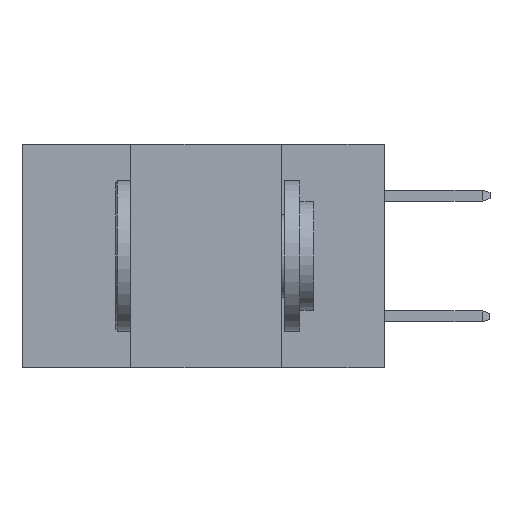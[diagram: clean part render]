
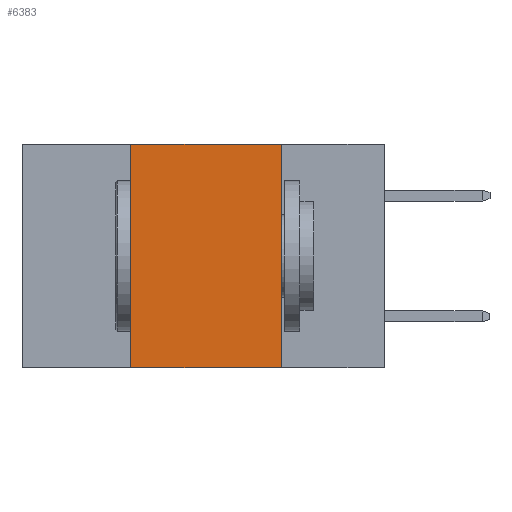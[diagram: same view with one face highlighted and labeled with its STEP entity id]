
A CAD part, left-side view. The second image highlights one B-rep face of the part: STEP entity #6383.
In plain terms, the highlighted planar face has unit normal (-1, 0, 0).
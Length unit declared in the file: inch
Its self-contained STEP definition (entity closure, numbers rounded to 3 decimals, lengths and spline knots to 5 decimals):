
#895 = CARTESIAN_POINT ( 'NONE',  ( 0., 0.17, 0. ) ) ;
#4665 = VECTOR ( 'NONE', #22252, 39.37008 ) ;
#5161 = EDGE_CURVE ( 'NONE', #11860, #26201, #27916, .T. ) ;
#5984 = CARTESIAN_POINT ( 'NONE',  ( 0., 0.6, 0. ) ) ;
#6094 = DIRECTION ( 'NONE',  ( 0., 0., -1. ) ) ;
#6383 = ADVANCED_FACE ( 'NONE', ( #26870 ), #7602, .F. ) ;
#7602 = PLANE ( 'NONE',  #23580 ) ;
#10028 = LINE ( 'NONE', #29526, #26945 ) ;
#10210 = VERTEX_POINT ( 'NONE', #15011 ) ;
#11301 = EDGE_LOOP ( 'NONE', ( #18695, #13994, #26219, #20837 ) ) ;
#11860 = VERTEX_POINT ( 'NONE', #23051 ) ;
#12345 = CARTESIAN_POINT ( 'NONE',  ( 0., 0.6, 0. ) ) ;
#13872 = EDGE_CURVE ( 'NONE', #10210, #11860, #20345, .T. ) ;
#13994 = ORIENTED_EDGE ( 'NONE', *, *, #5161, .F. ) ;
#14109 = CARTESIAN_POINT ( 'NONE',  ( 0., 0.42, 0. ) ) ;
#14676 = DIRECTION ( 'NONE',  ( 0., 0., -1. ) ) ;
#14874 = VECTOR ( 'NONE', #6094, 39.37008 ) ;
#15011 = CARTESIAN_POINT ( 'NONE',  ( 0., 0.42, -0.37 ) ) ;
#17770 = CARTESIAN_POINT ( 'NONE',  ( 0., 0.17, 0. ) ) ;
#18568 = EDGE_CURVE ( 'NONE', #26201, #20128, #27071, .T. ) ;
#18695 = ORIENTED_EDGE ( 'NONE', *, *, #18568, .F. ) ;
#20021 = EDGE_CURVE ( 'NONE', #10210, #20128, #10028, .T. ) ;
#20128 = VERTEX_POINT ( 'NONE', #23087 ) ;
#20345 = LINE ( 'NONE', #14109, #25030 ) ;
#20370 = DIRECTION ( 'NONE',  ( 0., -1., 0. ) ) ;
#20837 = ORIENTED_EDGE ( 'NONE', *, *, #20021, .T. ) ;
#22252 = DIRECTION ( 'NONE',  ( 0., -1., 0. ) ) ;
#23051 = CARTESIAN_POINT ( 'NONE',  ( 0., 0.42, 0. ) ) ;
#23087 = CARTESIAN_POINT ( 'NONE',  ( 0., 0.17, -0.37 ) ) ;
#23580 = AXIS2_PLACEMENT_3D ( 'NONE', #12345, #28444, #14676 ) ;
#25030 = VECTOR ( 'NONE', #30207, 39.37008 ) ;
#26201 = VERTEX_POINT ( 'NONE', #895 ) ;
#26219 = ORIENTED_EDGE ( 'NONE', *, *, #13872, .F. ) ;
#26870 = FACE_OUTER_BOUND ( 'NONE', #11301, .T. ) ;
#26945 = VECTOR ( 'NONE', #20370, 39.37008 ) ;
#27071 = LINE ( 'NONE', #17770, #14874 ) ;
#27916 = LINE ( 'NONE', #5984, #4665 ) ;
#28444 = DIRECTION ( 'NONE',  ( 1., 0., 0. ) ) ;
#29526 = CARTESIAN_POINT ( 'NONE',  ( 0., 0.6, -0.37 ) ) ;
#30207 = DIRECTION ( 'NONE',  ( 0., 0., 1. ) ) ;
